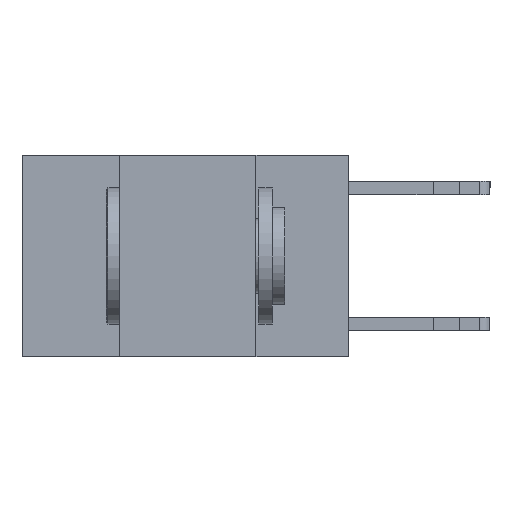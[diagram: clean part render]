
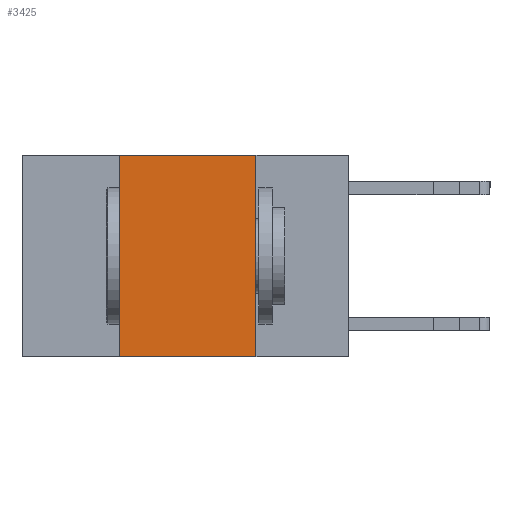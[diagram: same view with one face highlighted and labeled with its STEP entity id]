
A CAD part, left-side view. The second image highlights one B-rep face of the part: STEP entity #3425.
In plain terms, the highlighted planar face has unit normal (-1, 0, 0).
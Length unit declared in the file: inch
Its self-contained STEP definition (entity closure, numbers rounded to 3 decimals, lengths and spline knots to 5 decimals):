
#613 = CARTESIAN_POINT ( 'NONE',  ( 0., 0.42, -0.37 ) ) ;
#878 = ORIENTED_EDGE ( 'NONE', *, *, #3997, .F. ) ;
#1552 = CARTESIAN_POINT ( 'NONE',  ( 0., 0.17, -0.37 ) ) ;
#1623 = CARTESIAN_POINT ( 'NONE',  ( 0., 0.17, 0. ) ) ;
#1683 = EDGE_CURVE ( 'NONE', #9578, #13363, #9557, .T. ) ;
#1869 = CARTESIAN_POINT ( 'NONE',  ( 0., 0.42, 0. ) ) ;
#2971 = PLANE ( 'NONE',  #3246 ) ;
#3246 = AXIS2_PLACEMENT_3D ( 'NONE', #6940, #13879, #13781 ) ;
#3425 = ADVANCED_FACE ( 'NONE', ( #16369 ), #2971, .F. ) ;
#3805 = EDGE_LOOP ( 'NONE', ( #10837, #878, #16453, #5786 ) ) ;
#3846 = VECTOR ( 'NONE', #9256, 39.37008 ) ;
#3997 = EDGE_CURVE ( 'NONE', #13363, #16299, #7562, .T. ) ;
#5786 = ORIENTED_EDGE ( 'NONE', *, *, #8487, .T. ) ;
#6230 = CARTESIAN_POINT ( 'NONE',  ( 0., 0.6, 0. ) ) ;
#6940 = CARTESIAN_POINT ( 'NONE',  ( 0., 0.6, 0. ) ) ;
#7127 = VERTEX_POINT ( 'NONE', #1552 ) ;
#7562 = LINE ( 'NONE', #6230, #3846 ) ;
#8487 = EDGE_CURVE ( 'NONE', #9578, #7127, #8666, .T. ) ;
#8666 = LINE ( 'NONE', #8756, #15564 ) ;
#8756 = CARTESIAN_POINT ( 'NONE',  ( 0., 0.6, -0.37 ) ) ;
#9256 = DIRECTION ( 'NONE',  ( 0., -1., 0. ) ) ;
#9557 = LINE ( 'NONE', #15228, #9964 ) ;
#9578 = VERTEX_POINT ( 'NONE', #613 ) ;
#9820 = LINE ( 'NONE', #1623, #10929 ) ;
#9964 = VECTOR ( 'NONE', #13715, 39.37008 ) ;
#10837 = ORIENTED_EDGE ( 'NONE', *, *, #14293, .F. ) ;
#10929 = VECTOR ( 'NONE', #16484, 39.37008 ) ;
#12860 = CARTESIAN_POINT ( 'NONE',  ( 0., 0.17, 0. ) ) ;
#13363 = VERTEX_POINT ( 'NONE', #1869 ) ;
#13715 = DIRECTION ( 'NONE',  ( 0., 0., 1. ) ) ;
#13781 = DIRECTION ( 'NONE',  ( 0., 0., -1. ) ) ;
#13879 = DIRECTION ( 'NONE',  ( 1., 0., 0. ) ) ;
#14020 = DIRECTION ( 'NONE',  ( 0., -1., 0. ) ) ;
#14293 = EDGE_CURVE ( 'NONE', #16299, #7127, #9820, .T. ) ;
#15228 = CARTESIAN_POINT ( 'NONE',  ( 0., 0.42, 0. ) ) ;
#15564 = VECTOR ( 'NONE', #14020, 39.37008 ) ;
#16299 = VERTEX_POINT ( 'NONE', #12860 ) ;
#16369 = FACE_OUTER_BOUND ( 'NONE', #3805, .T. ) ;
#16453 = ORIENTED_EDGE ( 'NONE', *, *, #1683, .F. ) ;
#16484 = DIRECTION ( 'NONE',  ( 0., 0., -1. ) ) ;
